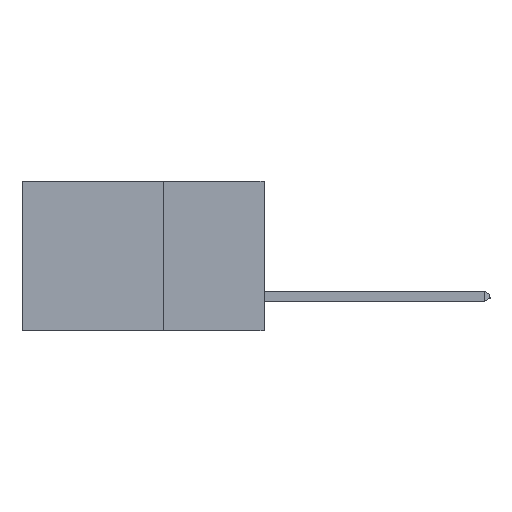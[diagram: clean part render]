
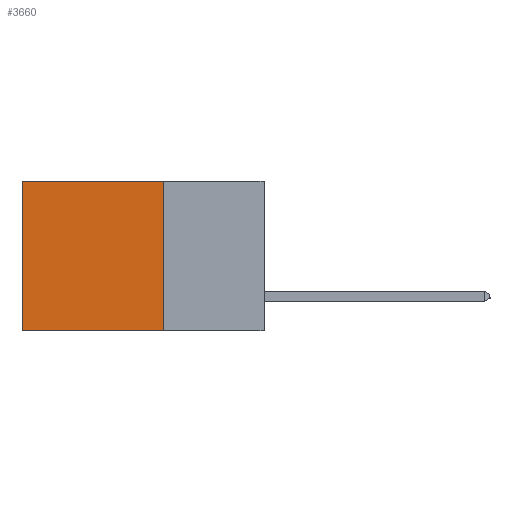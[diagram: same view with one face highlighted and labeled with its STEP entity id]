
A CAD part, left-side view. The second image highlights one B-rep face of the part: STEP entity #3660.
In plain terms, the highlighted planar face has unit normal (-1, 0, 0).
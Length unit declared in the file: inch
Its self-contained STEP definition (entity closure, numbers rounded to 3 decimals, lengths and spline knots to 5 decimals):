
#840 = VERTEX_POINT ( 'NONE', #3347 ) ;
#985 = CARTESIAN_POINT ( 'NONE',  ( 0.298, 0.6, 0. ) ) ;
#1159 = ORIENTED_EDGE ( 'NONE', *, *, #9733, .F. ) ;
#1284 = VERTEX_POINT ( 'NONE', #10326 ) ;
#1543 = LINE ( 'NONE', #4835, #6481 ) ;
#1975 = EDGE_CURVE ( 'NONE', #840, #3763, #1543, .T. ) ;
#2442 = ORIENTED_EDGE ( 'NONE', *, *, #8270, .F. ) ;
#3118 = DIRECTION ( 'NONE',  ( 0., 0., -1. ) ) ;
#3347 = CARTESIAN_POINT ( 'NONE',  ( 0.298, 0.25, 0. ) ) ;
#3660 = ADVANCED_FACE ( 'NONE', ( #11114 ), #10639, .F. ) ;
#3763 = VERTEX_POINT ( 'NONE', #10784 ) ;
#4061 = CARTESIAN_POINT ( 'NONE',  ( 0.298, 0.25, 0. ) ) ;
#4155 = VECTOR ( 'NONE', #8532, 39.37008 ) ;
#4473 = VECTOR ( 'NONE', #5922, 39.37008 ) ;
#4835 = CARTESIAN_POINT ( 'NONE',  ( 0.298, 0.25, 0. ) ) ;
#5679 = AXIS2_PLACEMENT_3D ( 'NONE', #4061, #11456, #6052 ) ;
#5823 = VERTEX_POINT ( 'NONE', #6254 ) ;
#5922 = DIRECTION ( 'NONE',  ( 0., 0., -1. ) ) ;
#6052 = DIRECTION ( 'NONE',  ( 0., 0., -1. ) ) ;
#6182 = EDGE_LOOP ( 'NONE', ( #11093, #1159, #2442, #11500 ) ) ;
#6254 = CARTESIAN_POINT ( 'NONE',  ( 0.298, 0.6, -0.37 ) ) ;
#6481 = VECTOR ( 'NONE', #8111, 39.37008 ) ;
#6658 = CARTESIAN_POINT ( 'NONE',  ( 0.298, 0.25, -0.37 ) ) ;
#6790 = LINE ( 'NONE', #8918, #9004 ) ;
#7075 = LINE ( 'NONE', #6658, #4155 ) ;
#8111 = DIRECTION ( 'NONE',  ( 0., 1., 0. ) ) ;
#8270 = EDGE_CURVE ( 'NONE', #840, #1284, #6790, .T. ) ;
#8532 = DIRECTION ( 'NONE',  ( 0., 1., 0. ) ) ;
#8918 = CARTESIAN_POINT ( 'NONE',  ( 0.298, 0.25, 0. ) ) ;
#9004 = VECTOR ( 'NONE', #3118, 39.37008 ) ;
#9297 = EDGE_CURVE ( 'NONE', #3763, #5823, #9559, .T. ) ;
#9559 = LINE ( 'NONE', #985, #4473 ) ;
#9733 = EDGE_CURVE ( 'NONE', #1284, #5823, #7075, .T. ) ;
#10326 = CARTESIAN_POINT ( 'NONE',  ( 0.298, 0.25, -0.37 ) ) ;
#10639 = PLANE ( 'NONE',  #5679 ) ;
#10784 = CARTESIAN_POINT ( 'NONE',  ( 0.298, 0.6, 0. ) ) ;
#11093 = ORIENTED_EDGE ( 'NONE', *, *, #9297, .T. ) ;
#11114 = FACE_OUTER_BOUND ( 'NONE', #6182, .T. ) ;
#11456 = DIRECTION ( 'NONE',  ( 1., 0., 0. ) ) ;
#11500 = ORIENTED_EDGE ( 'NONE', *, *, #1975, .T. ) ;
